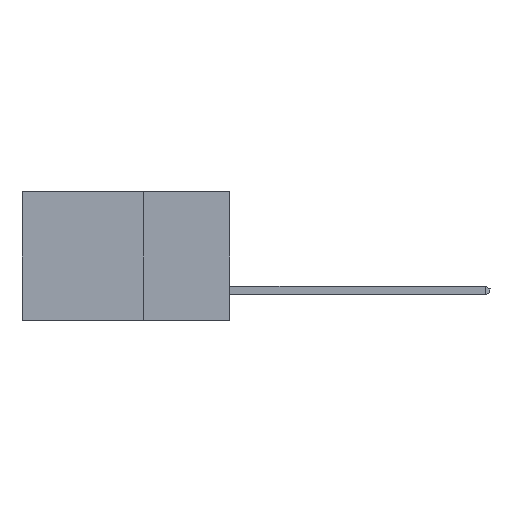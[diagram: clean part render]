
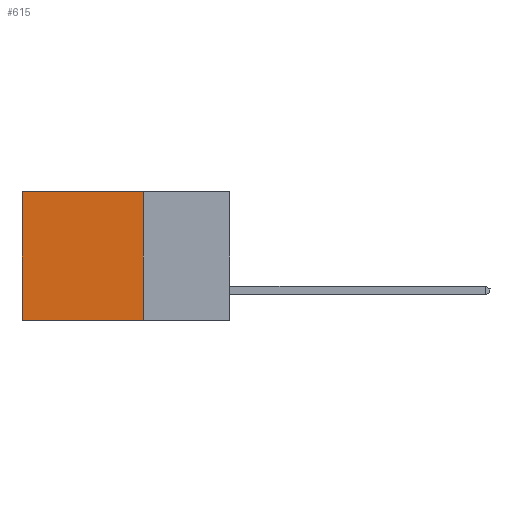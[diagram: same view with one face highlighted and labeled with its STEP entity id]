
A CAD part, left-side view. The second image highlights one B-rep face of the part: STEP entity #615.
In plain terms, the highlighted planar face has unit normal (-1, 0, 0).
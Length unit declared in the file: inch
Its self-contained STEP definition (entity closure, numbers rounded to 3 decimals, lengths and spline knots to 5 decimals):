
#85 = VERTEX_POINT ( 'NONE', #9517 ) ;
#276 = DIRECTION ( 'NONE',  ( 0., 0., -1. ) ) ;
#289 = DIRECTION ( 'NONE',  ( 0., 0., -1. ) ) ;
#447 = EDGE_LOOP ( 'NONE', ( #3895, #4680, #3006, #999 ) ) ;
#615 = ADVANCED_FACE ( 'NONE', ( #8585 ), #4012, .F. ) ;
#616 = VECTOR ( 'NONE', #3104, 39.37008 ) ;
#944 = VECTOR ( 'NONE', #3348, 39.37008 ) ;
#999 = ORIENTED_EDGE ( 'NONE', *, *, #3031, .T. ) ;
#1116 = VECTOR ( 'NONE', #5115, 39.37008 ) ;
#1123 = CARTESIAN_POINT ( 'NONE',  ( 0.2615, 0.6, -0.37 ) ) ;
#1124 = EDGE_CURVE ( 'NONE', #5817, #85, #3950, .T. ) ;
#1936 = EDGE_CURVE ( 'NONE', #85, #3127, #3152, .T. ) ;
#3006 = ORIENTED_EDGE ( 'NONE', *, *, #1124, .F. ) ;
#3031 = EDGE_CURVE ( 'NONE', #5817, #7302, #7481, .T. ) ;
#3104 = DIRECTION ( 'NONE',  ( 0., 1., 0. ) ) ;
#3127 = VERTEX_POINT ( 'NONE', #4777 ) ;
#3152 = LINE ( 'NONE', #9084, #616 ) ;
#3348 = DIRECTION ( 'NONE',  ( 0., 0., -1. ) ) ;
#3540 = CARTESIAN_POINT ( 'NONE',  ( 0.2615, 0.25, 0. ) ) ;
#3784 = EDGE_CURVE ( 'NONE', #7302, #3127, #4960, .T. ) ;
#3895 = ORIENTED_EDGE ( 'NONE', *, *, #3784, .T. ) ;
#3950 = LINE ( 'NONE', #6314, #6970 ) ;
#4012 = PLANE ( 'NONE',  #5572 ) ;
#4521 = CARTESIAN_POINT ( 'NONE',  ( 0.2615, 0.25, 0. ) ) ;
#4680 = ORIENTED_EDGE ( 'NONE', *, *, #1936, .F. ) ;
#4777 = CARTESIAN_POINT ( 'NONE',  ( 0.2615, 0.6, -0.37 ) ) ;
#4859 = DIRECTION ( 'NONE',  ( 1., 0., 0. ) ) ;
#4960 = LINE ( 'NONE', #1123, #944 ) ;
#5115 = DIRECTION ( 'NONE',  ( 0., 1., 0. ) ) ;
#5572 = AXIS2_PLACEMENT_3D ( 'NONE', #6944, #4859, #289 ) ;
#5817 = VERTEX_POINT ( 'NONE', #3540 ) ;
#6117 = CARTESIAN_POINT ( 'NONE',  ( 0.2615, 0.6, 0. ) ) ;
#6314 = CARTESIAN_POINT ( 'NONE',  ( 0.2615, 0.25, -0.37 ) ) ;
#6944 = CARTESIAN_POINT ( 'NONE',  ( 0.2615, 0.25, -0.37 ) ) ;
#6970 = VECTOR ( 'NONE', #276, 39.37008 ) ;
#7302 = VERTEX_POINT ( 'NONE', #6117 ) ;
#7481 = LINE ( 'NONE', #4521, #1116 ) ;
#8585 = FACE_OUTER_BOUND ( 'NONE', #447, .T. ) ;
#9084 = CARTESIAN_POINT ( 'NONE',  ( 0.2615, 0.25, -0.37 ) ) ;
#9517 = CARTESIAN_POINT ( 'NONE',  ( 0.2615, 0.25, -0.37 ) ) ;
